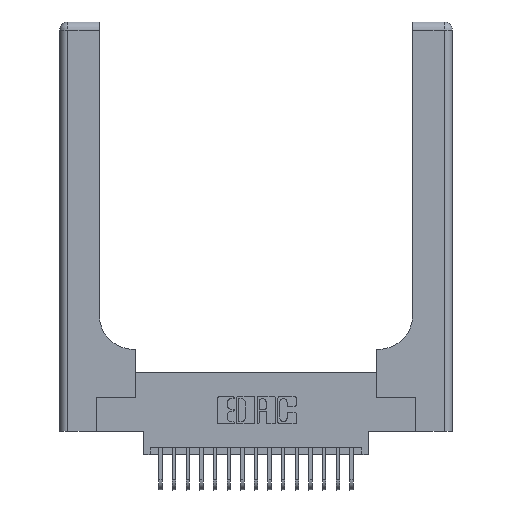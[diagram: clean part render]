
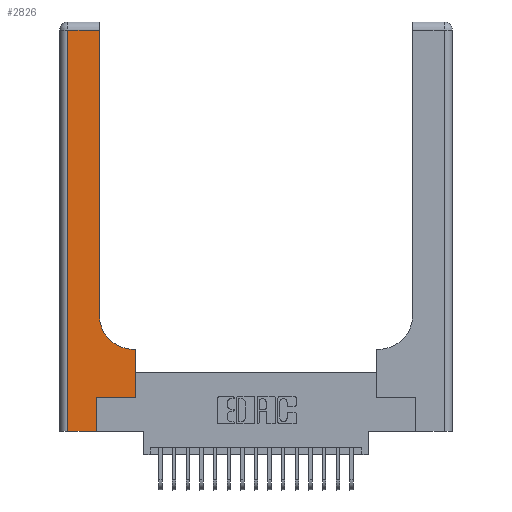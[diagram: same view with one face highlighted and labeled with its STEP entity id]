
A CAD part, top view. The second image highlights one B-rep face of the part: STEP entity #2826.
In plain terms, the highlighted planar face has unit normal (0, 0, 1).
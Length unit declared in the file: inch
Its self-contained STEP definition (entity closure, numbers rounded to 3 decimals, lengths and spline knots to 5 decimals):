
#332 = EDGE_CURVE ( 'NONE', #21698, #15941, #16862, .T. ) ;
#1206 = CARTESIAN_POINT ( 'NONE',  ( 0.269, 0., 0.37 ) ) ;
#1393 = CARTESIAN_POINT ( 'NONE',  ( 0.2915, 3., 0.37 ) ) ;
#1775 = ORIENTED_EDGE ( 'NONE', *, *, #14563, .T. ) ;
#1854 = VERTEX_POINT ( 'NONE', #5029 ) ;
#1882 = EDGE_CURVE ( 'NONE', #2449, #13913, #15007, .T. ) ;
#2181 = VECTOR ( 'NONE', #21118, 39.37008 ) ;
#2449 = VERTEX_POINT ( 'NONE', #20534 ) ;
#2461 = LINE ( 'NONE', #14819, #6527 ) ;
#2562 = CIRCLE ( 'NONE', #9123, 0.25 ) ;
#2826 = ADVANCED_FACE ( 'NONE', ( #3344 ), #18894, .F. ) ;
#3113 = CARTESIAN_POINT ( 'NONE',  ( 0.06, 3., 0.37 ) ) ;
#3294 = DIRECTION ( 'NONE',  ( 0., 0., -1. ) ) ;
#3319 = ORIENTED_EDGE ( 'NONE', *, *, #13520, .T. ) ;
#3344 = FACE_OUTER_BOUND ( 'NONE', #19200, .T. ) ;
#4056 = CARTESIAN_POINT ( 'NONE',  ( 0., 0., 0.37 ) ) ;
#4843 = EDGE_CURVE ( 'NONE', #10437, #21698, #11124, .T. ) ;
#5019 = EDGE_CURVE ( 'NONE', #13261, #10437, #2461, .T. ) ;
#5029 = CARTESIAN_POINT ( 'NONE',  ( 0.2915, 2.94, 0.37 ) ) ;
#5273 = DIRECTION ( 'NONE',  ( 1., 0., 0. ) ) ;
#6145 = CARTESIAN_POINT ( 'NONE',  ( 0.269, 0., 0.37 ) ) ;
#6380 = LINE ( 'NONE', #1393, #13670 ) ;
#6527 = VECTOR ( 'NONE', #14897, 39.37008 ) ;
#6573 = CARTESIAN_POINT ( 'NONE',  ( 0.5585, 0.25, 0.37 ) ) ;
#6735 = CARTESIAN_POINT ( 'NONE',  ( 0.06, 0., 0.37 ) ) ;
#7868 = DIRECTION ( 'NONE',  ( 0., 1., 0. ) ) ;
#8655 = CARTESIAN_POINT ( 'NONE',  ( 0.269, 0.25, 0.37 ) ) ;
#9123 = AXIS2_PLACEMENT_3D ( 'NONE', #15637, #3294, #5273 ) ;
#9553 = ORIENTED_EDGE ( 'NONE', *, *, #1882, .T. ) ;
#9706 = ORIENTED_EDGE ( 'NONE', *, *, #4843, .T. ) ;
#9772 = DIRECTION ( 'NONE',  ( -1., 0., 0. ) ) ;
#9867 = ORIENTED_EDGE ( 'NONE', *, *, #332, .T. ) ;
#10168 = VECTOR ( 'NONE', #14246, 39.37008 ) ;
#10372 = DIRECTION ( 'NONE',  ( -1., 0., 0. ) ) ;
#10437 = VERTEX_POINT ( 'NONE', #6573 ) ;
#11124 = LINE ( 'NONE', #21046, #2181 ) ;
#12071 = ORIENTED_EDGE ( 'NONE', *, *, #5019, .T. ) ;
#12292 = VECTOR ( 'NONE', #9772, 39.37008 ) ;
#12613 = VERTEX_POINT ( 'NONE', #13293 ) ;
#13261 = VERTEX_POINT ( 'NONE', #8655 ) ;
#13293 = CARTESIAN_POINT ( 'NONE',  ( 0.2915, 0.85, 0.37 ) ) ;
#13520 = EDGE_CURVE ( 'NONE', #13913, #13721, #18803, .T. ) ;
#13670 = VECTOR ( 'NONE', #15250, 39.37008 ) ;
#13721 = VERTEX_POINT ( 'NONE', #1206 ) ;
#13795 = ORIENTED_EDGE ( 'NONE', *, *, #13986, .T. ) ;
#13913 = VERTEX_POINT ( 'NONE', #6735 ) ;
#13986 = EDGE_CURVE ( 'NONE', #1854, #2449, #14517, .T. ) ;
#14246 = DIRECTION ( 'NONE',  ( 1., 0., 0. ) ) ;
#14255 = VECTOR ( 'NONE', #15591, 39.37008 ) ;
#14478 = VECTOR ( 'NONE', #18617, 39.37008 ) ;
#14517 = LINE ( 'NONE', #17221, #14255 ) ;
#14563 = EDGE_CURVE ( 'NONE', #15941, #12613, #2562, .T. ) ;
#14819 = CARTESIAN_POINT ( 'NONE',  ( 0.269, 0.25, 0.37 ) ) ;
#14897 = DIRECTION ( 'NONE',  ( 1., 0., 0. ) ) ;
#15007 = LINE ( 'NONE', #3113, #14478 ) ;
#15250 = DIRECTION ( 'NONE',  ( 0., 1., 0. ) ) ;
#15591 = DIRECTION ( 'NONE',  ( -1., 0., 0. ) ) ;
#15606 = VECTOR ( 'NONE', #7868, 39.37008 ) ;
#15637 = CARTESIAN_POINT ( 'NONE',  ( 0.5415, 0.85, 0.37 ) ) ;
#15906 = AXIS2_PLACEMENT_3D ( 'NONE', #20646, #22209, #10372 ) ;
#15941 = VERTEX_POINT ( 'NONE', #21752 ) ;
#16862 = LINE ( 'NONE', #20053, #12292 ) ;
#17221 = CARTESIAN_POINT ( 'NONE',  ( 0., 2.94, 0.37 ) ) ;
#17763 = LINE ( 'NONE', #6145, #15606 ) ;
#18617 = DIRECTION ( 'NONE',  ( 0., -1., 0. ) ) ;
#18715 = ORIENTED_EDGE ( 'NONE', *, *, #20725, .T. ) ;
#18803 = LINE ( 'NONE', #4056, #10168 ) ;
#18894 = PLANE ( 'NONE',  #15906 ) ;
#19200 = EDGE_LOOP ( 'NONE', ( #18715, #13795, #9553, #3319, #21082, #12071, #9706, #9867, #1775 ) ) ;
#20004 = EDGE_CURVE ( 'NONE', #13721, #13261, #17763, .T. ) ;
#20053 = CARTESIAN_POINT ( 'NONE',  ( 0.2915, 0.6, 0.37 ) ) ;
#20534 = CARTESIAN_POINT ( 'NONE',  ( 0.06, 2.94, 0.37 ) ) ;
#20646 = CARTESIAN_POINT ( 'NONE',  ( 0., 3., 0.37 ) ) ;
#20725 = EDGE_CURVE ( 'NONE', #12613, #1854, #6380, .T. ) ;
#21046 = CARTESIAN_POINT ( 'NONE',  ( 0.5585, 0.25, 0.37 ) ) ;
#21082 = ORIENTED_EDGE ( 'NONE', *, *, #20004, .T. ) ;
#21118 = DIRECTION ( 'NONE',  ( 0., 1., 0. ) ) ;
#21698 = VERTEX_POINT ( 'NONE', #22389 ) ;
#21752 = CARTESIAN_POINT ( 'NONE',  ( 0.5415, 0.6, 0.37 ) ) ;
#22209 = DIRECTION ( 'NONE',  ( 0., 0., -1. ) ) ;
#22389 = CARTESIAN_POINT ( 'NONE',  ( 0.5585, 0.6, 0.37 ) ) ;
